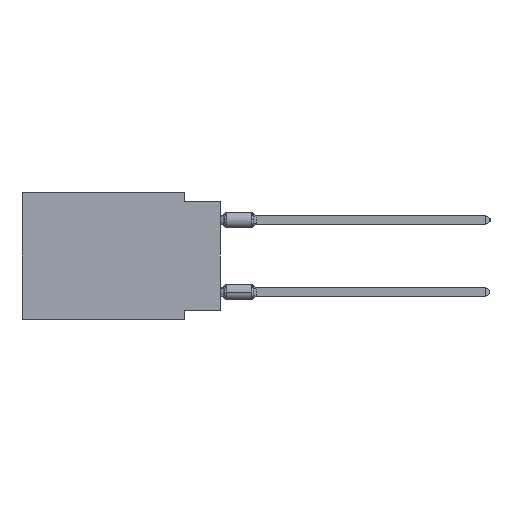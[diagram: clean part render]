
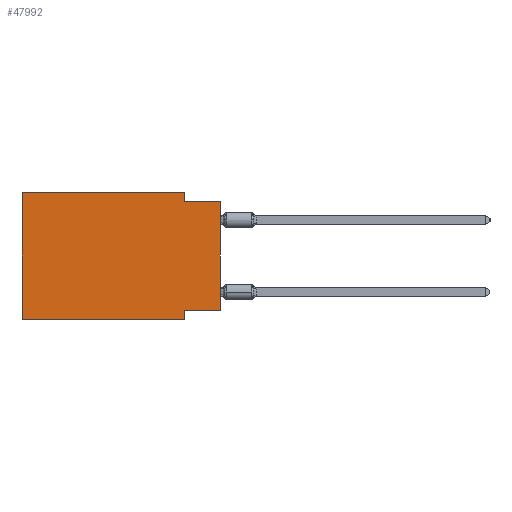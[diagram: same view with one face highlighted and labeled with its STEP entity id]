
A CAD part, left-side view. The second image highlights one B-rep face of the part: STEP entity #47992.
In plain terms, the highlighted planar face has unit normal (-1, 0, 0).
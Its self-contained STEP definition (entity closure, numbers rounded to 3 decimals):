
#296 = CARTESIAN_POINT ( 'NONE',  ( 0., 0., -8.255 ) ) ;
#833 = LINE ( 'NONE', #35834, #46044 ) ;
#935 = CARTESIAN_POINT ( 'NONE',  ( 0., 13.97, 0. ) ) ;
#1635 = VERTEX_POINT ( 'NONE', #42629 ) ;
#2368 = CARTESIAN_POINT ( 'NONE',  ( 0., 0., 0. ) ) ;
#2630 = VERTEX_POINT ( 'NONE', #42765 ) ;
#2750 = CARTESIAN_POINT ( 'NONE',  ( 0., 13.97, -8.89 ) ) ;
#3552 = CARTESIAN_POINT ( 'NONE',  ( 0., 0., -8.255 ) ) ;
#4671 = VERTEX_POINT ( 'NONE', #2750 ) ;
#4809 = VERTEX_POINT ( 'NONE', #21205 ) ;
#7586 = AXIS2_PLACEMENT_3D ( 'NONE', #38908, #42904, #29538 ) ;
#10587 = LINE ( 'NONE', #41018, #55249 ) ;
#10711 = VECTOR ( 'NONE', #55364, 1000. ) ;
#11925 = ORIENTED_EDGE ( 'NONE', *, *, #40795, .F. ) ;
#12245 = VERTEX_POINT ( 'NONE', #22368 ) ;
#12762 = ORIENTED_EDGE ( 'NONE', *, *, #54863, .F. ) ;
#13406 = CARTESIAN_POINT ( 'NONE',  ( 0., 2.54, 0. ) ) ;
#14092 = EDGE_CURVE ( 'NONE', #26265, #1635, #47007, .T. ) ;
#14771 = VERTEX_POINT ( 'NONE', #935 ) ;
#17254 = DIRECTION ( 'NONE',  ( 0., -1., 0. ) ) ;
#19342 = ORIENTED_EDGE ( 'NONE', *, *, #37485, .T. ) ;
#21205 = CARTESIAN_POINT ( 'NONE',  ( 0., 2.54, -0.635 ) ) ;
#22211 = DIRECTION ( 'NONE',  ( 0., 0., -1. ) ) ;
#22280 = CARTESIAN_POINT ( 'NONE',  ( 0., 2.54, -8.89 ) ) ;
#22368 = CARTESIAN_POINT ( 'NONE',  ( 0., 2.54, 0. ) ) ;
#23410 = LINE ( 'NONE', #2368, #43884 ) ;
#25860 = VECTOR ( 'NONE', #45042, 1000. ) ;
#25935 = DIRECTION ( 'NONE',  ( 0., 1., 0. ) ) ;
#26265 = VERTEX_POINT ( 'NONE', #3552 ) ;
#27017 = DIRECTION ( 'NONE',  ( 0., -1., 0. ) ) ;
#27358 = DIRECTION ( 'NONE',  ( 0., -1., 0. ) ) ;
#27653 = ORIENTED_EDGE ( 'NONE', *, *, #41155, .F. ) ;
#28608 = VECTOR ( 'NONE', #22211, 1000. ) ;
#29527 = CARTESIAN_POINT ( 'NONE',  ( 0., 13.97, -8.89 ) ) ;
#29538 = DIRECTION ( 'NONE',  ( 0., 0., -1. ) ) ;
#31608 = LINE ( 'NONE', #13406, #28608 ) ;
#31942 = LINE ( 'NONE', #22280, #25860 ) ;
#32096 = VECTOR ( 'NONE', #25935, 1000. ) ;
#32838 = VECTOR ( 'NONE', #17254, 1000. ) ;
#33177 = EDGE_CURVE ( 'NONE', #4671, #35374, #33529, .T. ) ;
#33338 = EDGE_LOOP ( 'NONE', ( #19342, #40338, #27653, #51398, #12762, #36458, #11925, #50579 ) ) ;
#33483 = LINE ( 'NONE', #45999, #10711 ) ;
#33529 = LINE ( 'NONE', #29527, #32838 ) ;
#35374 = VERTEX_POINT ( 'NONE', #49126 ) ;
#35834 = CARTESIAN_POINT ( 'NONE',  ( 0., 13.97, 0. ) ) ;
#36458 = ORIENTED_EDGE ( 'NONE', *, *, #33177, .T. ) ;
#37485 = EDGE_CURVE ( 'NONE', #26265, #2630, #23410, .T. ) ;
#38908 = CARTESIAN_POINT ( 'NONE',  ( 0., 13.97, 0. ) ) ;
#40338 = ORIENTED_EDGE ( 'NONE', *, *, #55461, .F. ) ;
#40795 = EDGE_CURVE ( 'NONE', #1635, #35374, #31942, .T. ) ;
#41018 = CARTESIAN_POINT ( 'NONE',  ( 0., 0., -0.635 ) ) ;
#41155 = EDGE_CURVE ( 'NONE', #12245, #4809, #31608, .T. ) ;
#42629 = CARTESIAN_POINT ( 'NONE',  ( 0., 2.54, -8.255 ) ) ;
#42765 = CARTESIAN_POINT ( 'NONE',  ( 0., 0., -0.635 ) ) ;
#42904 = DIRECTION ( 'NONE',  ( 1., 0., 0. ) ) ;
#43884 = VECTOR ( 'NONE', #54681, 1000. ) ;
#45042 = DIRECTION ( 'NONE',  ( 0., 0., -1. ) ) ;
#45999 = CARTESIAN_POINT ( 'NONE',  ( 0., 13.97, 0. ) ) ;
#46044 = VECTOR ( 'NONE', #27017, 1000. ) ;
#46602 = PLANE ( 'NONE',  #7586 ) ;
#47007 = LINE ( 'NONE', #296, #32096 ) ;
#47992 = ADVANCED_FACE ( 'NONE', ( #55695 ), #46602, .F. ) ;
#49126 = CARTESIAN_POINT ( 'NONE',  ( 0., 2.54, -8.89 ) ) ;
#50579 = ORIENTED_EDGE ( 'NONE', *, *, #14092, .F. ) ;
#51398 = ORIENTED_EDGE ( 'NONE', *, *, #53649, .F. ) ;
#53649 = EDGE_CURVE ( 'NONE', #14771, #12245, #833, .T. ) ;
#54681 = DIRECTION ( 'NONE',  ( 0., 0., 1. ) ) ;
#54863 = EDGE_CURVE ( 'NONE', #4671, #14771, #33483, .T. ) ;
#55249 = VECTOR ( 'NONE', #27358, 1000. ) ;
#55364 = DIRECTION ( 'NONE',  ( 0., 0., 1. ) ) ;
#55461 = EDGE_CURVE ( 'NONE', #4809, #2630, #10587, .T. ) ;
#55695 = FACE_OUTER_BOUND ( 'NONE', #33338, .T. ) ;
